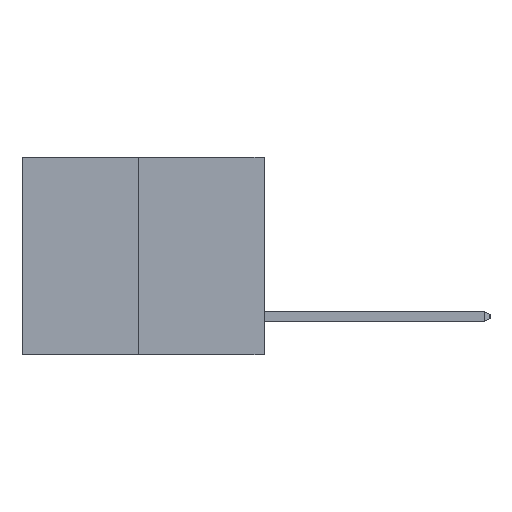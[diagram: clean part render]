
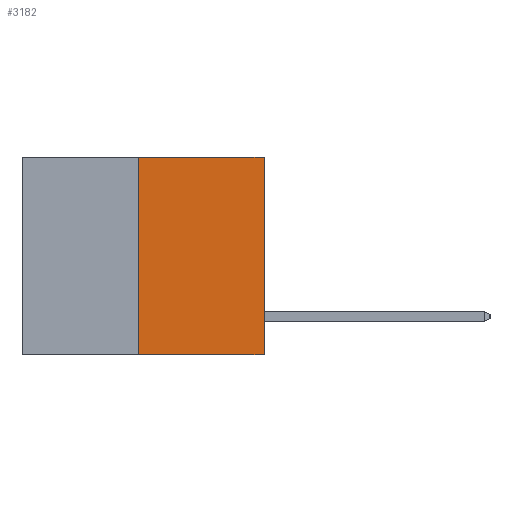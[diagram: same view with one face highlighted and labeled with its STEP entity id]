
A CAD part, left-side view. The second image highlights one B-rep face of the part: STEP entity #3182.
In plain terms, the highlighted planar face has unit normal (-1, 0, 0).
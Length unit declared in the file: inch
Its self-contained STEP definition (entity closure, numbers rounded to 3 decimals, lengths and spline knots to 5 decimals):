
#332 = CARTESIAN_POINT ( 'NONE',  ( 0., 0.6, -0.49 ) ) ;
#889 = LINE ( 'NONE', #332, #8180 ) ;
#944 = PLANE ( 'NONE',  #3288 ) ;
#1056 = ORIENTED_EDGE ( 'NONE', *, *, #12708, .F. ) ;
#1070 = DIRECTION ( 'NONE',  ( 0., 0., 1. ) ) ;
#1254 = VERTEX_POINT ( 'NONE', #10955 ) ;
#1749 = CARTESIAN_POINT ( 'NONE',  ( 0., 0.6, 0. ) ) ;
#1783 = LINE ( 'NONE', #3513, #4736 ) ;
#2055 = DIRECTION ( 'NONE',  ( 1., 0., 0. ) ) ;
#2630 = LINE ( 'NONE', #3444, #11143 ) ;
#3083 = EDGE_LOOP ( 'NONE', ( #3276, #6823, #5544, #1056 ) ) ;
#3164 = DIRECTION ( 'NONE',  ( 0., 0., -1. ) ) ;
#3182 = ADVANCED_FACE ( 'NONE', ( #5520 ), #944, .F. ) ;
#3276 = ORIENTED_EDGE ( 'NONE', *, *, #6606, .F. ) ;
#3288 = AXIS2_PLACEMENT_3D ( 'NONE', #9781, #2055, #3164 ) ;
#3444 = CARTESIAN_POINT ( 'NONE',  ( 0., 0., 0. ) ) ;
#3448 = VERTEX_POINT ( 'NONE', #6417 ) ;
#3513 = CARTESIAN_POINT ( 'NONE',  ( 0., 0.312, -0.49 ) ) ;
#4181 = VERTEX_POINT ( 'NONE', #13622 ) ;
#4736 = VECTOR ( 'NONE', #10140, 39.37008 ) ;
#4867 = LINE ( 'NONE', #1749, #11100 ) ;
#5515 = CARTESIAN_POINT ( 'NONE',  ( 0., 0.312, 0. ) ) ;
#5520 = FACE_OUTER_BOUND ( 'NONE', #3083, .T. ) ;
#5544 = ORIENTED_EDGE ( 'NONE', *, *, #10555, .T. ) ;
#6417 = CARTESIAN_POINT ( 'NONE',  ( 0., 0., 0. ) ) ;
#6606 = EDGE_CURVE ( 'NONE', #1254, #6933, #1783, .T. ) ;
#6823 = ORIENTED_EDGE ( 'NONE', *, *, #7265, .T. ) ;
#6933 = VERTEX_POINT ( 'NONE', #5515 ) ;
#6946 = DIRECTION ( 'NONE',  ( 0., -1., 0. ) ) ;
#7265 = EDGE_CURVE ( 'NONE', #1254, #4181, #889, .T. ) ;
#8180 = VECTOR ( 'NONE', #6946, 39.37008 ) ;
#9781 = CARTESIAN_POINT ( 'NONE',  ( 0., 0.6, 0. ) ) ;
#10140 = DIRECTION ( 'NONE',  ( 0., 0., 1. ) ) ;
#10543 = DIRECTION ( 'NONE',  ( 0., -1., 0. ) ) ;
#10555 = EDGE_CURVE ( 'NONE', #4181, #3448, #2630, .T. ) ;
#10955 = CARTESIAN_POINT ( 'NONE',  ( 0., 0.312, -0.49 ) ) ;
#11100 = VECTOR ( 'NONE', #10543, 39.37008 ) ;
#11143 = VECTOR ( 'NONE', #1070, 39.37008 ) ;
#12708 = EDGE_CURVE ( 'NONE', #6933, #3448, #4867, .T. ) ;
#13622 = CARTESIAN_POINT ( 'NONE',  ( 0., 0., -0.49 ) ) ;
